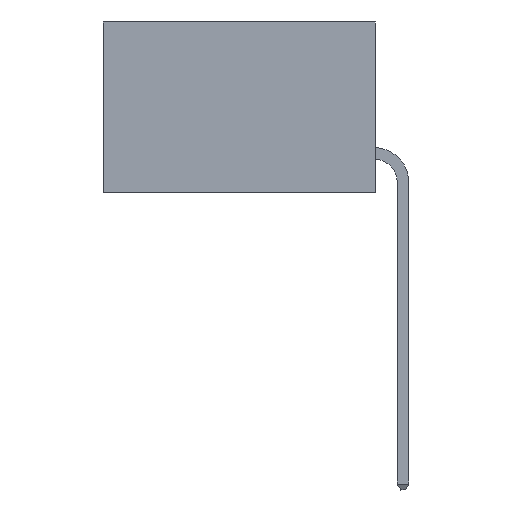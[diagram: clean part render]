
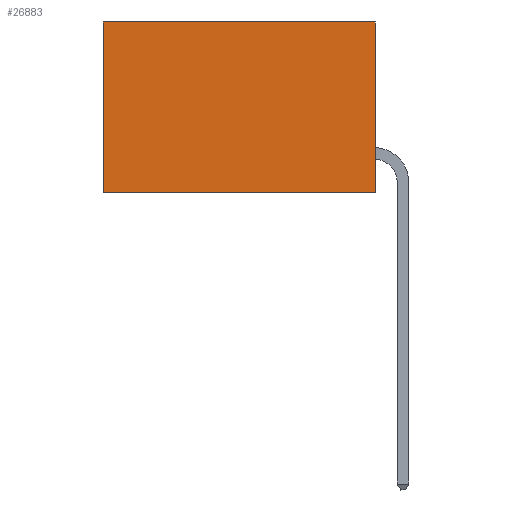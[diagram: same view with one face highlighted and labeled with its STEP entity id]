
A CAD part, left-side view. The second image highlights one B-rep face of the part: STEP entity #26883.
In plain terms, the highlighted planar face has unit normal (-1, 0, 0).
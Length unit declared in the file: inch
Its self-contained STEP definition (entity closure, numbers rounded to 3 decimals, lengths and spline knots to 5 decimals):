
#821 = VECTOR ( 'NONE', #13123, 39.37008 ) ;
#1080 = DIRECTION ( 'NONE',  ( 1., 0., 0. ) ) ;
#1182 = VERTEX_POINT ( 'NONE', #4974 ) ;
#2115 = AXIS2_PLACEMENT_3D ( 'NONE', #22688, #1080, #16266 ) ;
#2149 = VERTEX_POINT ( 'NONE', #3213 ) ;
#2218 = DIRECTION ( 'NONE',  ( 0., 1., 0. ) ) ;
#3213 = CARTESIAN_POINT ( 'NONE',  ( 0.277, 0., -0.37 ) ) ;
#4974 = CARTESIAN_POINT ( 'NONE',  ( 0.277, 0.59, -0.37 ) ) ;
#5951 = VERTEX_POINT ( 'NONE', #20857 ) ;
#6276 = VECTOR ( 'NONE', #25807, 39.37008 ) ;
#6328 = CARTESIAN_POINT ( 'NONE',  ( 0.277, 0.59, -0.37 ) ) ;
#8445 = CARTESIAN_POINT ( 'NONE',  ( 0.277, 0., 0. ) ) ;
#8547 = DIRECTION ( 'NONE',  ( 0., 1., 0. ) ) ;
#9586 = EDGE_CURVE ( 'NONE', #22369, #1182, #17838, .T. ) ;
#10146 = ORIENTED_EDGE ( 'NONE', *, *, #9586, .T. ) ;
#10465 = EDGE_CURVE ( 'NONE', #5951, #2149, #13068, .T. ) ;
#11462 = EDGE_CURVE ( 'NONE', #2149, #1182, #24289, .T. ) ;
#11557 = ORIENTED_EDGE ( 'NONE', *, *, #26514, .T. ) ;
#13068 = LINE ( 'NONE', #13361, #821 ) ;
#13072 = CARTESIAN_POINT ( 'NONE',  ( 0.277, 0.59, 0. ) ) ;
#13123 = DIRECTION ( 'NONE',  ( 0., 0., -1. ) ) ;
#13317 = VECTOR ( 'NONE', #8547, 39.37008 ) ;
#13361 = CARTESIAN_POINT ( 'NONE',  ( 0.277, 0., -0.37 ) ) ;
#16266 = DIRECTION ( 'NONE',  ( 0., 0., -1. ) ) ;
#17838 = LINE ( 'NONE', #6328, #6276 ) ;
#19143 = LINE ( 'NONE', #8445, #13317 ) ;
#19213 = CARTESIAN_POINT ( 'NONE',  ( 0.277, 0., -0.37 ) ) ;
#20857 = CARTESIAN_POINT ( 'NONE',  ( 0.277, 0., 0. ) ) ;
#22369 = VERTEX_POINT ( 'NONE', #13072 ) ;
#22688 = CARTESIAN_POINT ( 'NONE',  ( 0.277, 0., -0.37 ) ) ;
#22956 = EDGE_LOOP ( 'NONE', ( #10146, #26447, #25983, #11557 ) ) ;
#23603 = VECTOR ( 'NONE', #2218, 39.37008 ) ;
#24289 = LINE ( 'NONE', #19213, #23603 ) ;
#25807 = DIRECTION ( 'NONE',  ( 0., 0., -1. ) ) ;
#25983 = ORIENTED_EDGE ( 'NONE', *, *, #10465, .F. ) ;
#26292 = FACE_OUTER_BOUND ( 'NONE', #22956, .T. ) ;
#26447 = ORIENTED_EDGE ( 'NONE', *, *, #11462, .F. ) ;
#26514 = EDGE_CURVE ( 'NONE', #5951, #22369, #19143, .T. ) ;
#26883 = ADVANCED_FACE ( 'NONE', ( #26292 ), #27186, .F. ) ;
#27186 = PLANE ( 'NONE',  #2115 ) ;
